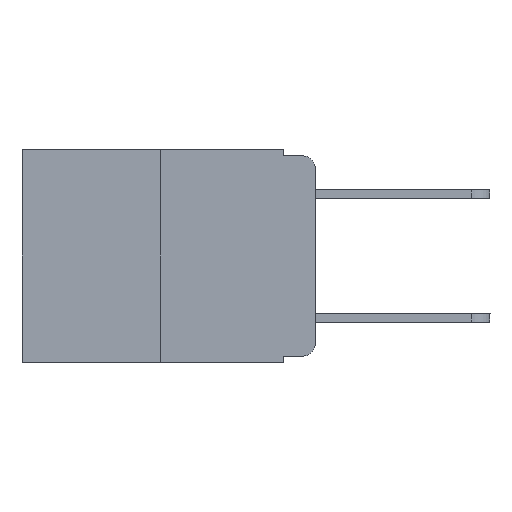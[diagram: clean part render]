
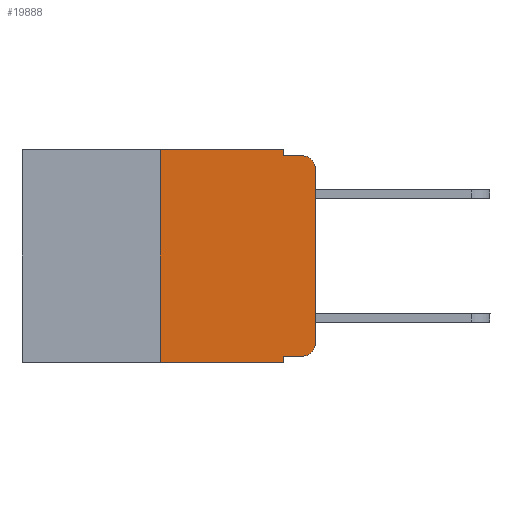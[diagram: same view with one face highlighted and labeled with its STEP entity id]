
A CAD part, left-side view. The second image highlights one B-rep face of the part: STEP entity #19888.
In plain terms, the highlighted planar face has unit normal (-1, 0, 0).
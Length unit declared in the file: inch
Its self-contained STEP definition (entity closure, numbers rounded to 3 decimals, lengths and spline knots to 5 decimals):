
#262 = VECTOR ( 'NONE', #478, 39.37008 ) ;
#307 = VECTOR ( 'NONE', #18379, 39.37008 ) ;
#478 = DIRECTION ( 'NONE',  ( 0., -1., 0. ) ) ;
#493 = DIRECTION ( 'NONE',  ( 0., 0., 1. ) ) ;
#509 = VECTOR ( 'NONE', #14346, 39.37008 ) ;
#698 = DIRECTION ( 'NONE',  ( 0., 0., -1. ) ) ;
#1296 = CARTESIAN_POINT ( 'NONE',  ( 0., 0.25, -0.343 ) ) ;
#1331 = CARTESIAN_POINT ( 'NONE',  ( 0., 0.051, 0. ) ) ;
#1610 = CIRCLE ( 'NONE', #6613, 0.02 ) ;
#1802 = VECTOR ( 'NONE', #15752, 39.37008 ) ;
#1815 = VECTOR ( 'NONE', #493, 39.37008 ) ;
#1986 = CARTESIAN_POINT ( 'NONE',  ( 0., 0.25, 0. ) ) ;
#2283 = CARTESIAN_POINT ( 'NONE',  ( 0., 0.02, -0.313 ) ) ;
#2319 = EDGE_CURVE ( 'NONE', #7240, #7508, #14245, .T. ) ;
#2642 = VERTEX_POINT ( 'NONE', #18880 ) ;
#3036 = ORIENTED_EDGE ( 'NONE', *, *, #4214, .F. ) ;
#3186 = CARTESIAN_POINT ( 'NONE',  ( 0., 0.473, -0.343 ) ) ;
#3391 = EDGE_LOOP ( 'NONE', ( #9204, #11643, #16425, #6075, #3036, #12622, #13894, #13338, #7596, #8342 ) ) ;
#3430 = EDGE_CURVE ( 'NONE', #6850, #14816, #12188, .T. ) ;
#3579 = VECTOR ( 'NONE', #698, 39.37008 ) ;
#3724 = LINE ( 'NONE', #6735, #509 ) ;
#3794 = LINE ( 'NONE', #6949, #1815 ) ;
#4214 = EDGE_CURVE ( 'NONE', #2642, #6850, #18089, .T. ) ;
#4427 = LINE ( 'NONE', #1986, #11347 ) ;
#5440 = EDGE_CURVE ( 'NONE', #14863, #7508, #12551, .T. ) ;
#5442 = CARTESIAN_POINT ( 'NONE',  ( 0., 0.473, 0. ) ) ;
#6024 = LINE ( 'NONE', #13960, #1802 ) ;
#6075 = ORIENTED_EDGE ( 'NONE', *, *, #3430, .F. ) ;
#6363 = AXIS2_PLACEMENT_3D ( 'NONE', #9629, #11213, #16265 ) ;
#6613 = AXIS2_PLACEMENT_3D ( 'NONE', #13531, #13325, #10352 ) ;
#6735 = CARTESIAN_POINT ( 'NONE',  ( 0., 0.051, -0.333 ) ) ;
#6784 = DIRECTION ( 'NONE',  ( 0., 0., 1. ) ) ;
#6850 = VERTEX_POINT ( 'NONE', #1331 ) ;
#6949 = CARTESIAN_POINT ( 'NONE',  ( 0., 0., 0. ) ) ;
#7031 = DIRECTION ( 'NONE',  ( 0., 0., -1. ) ) ;
#7192 = CARTESIAN_POINT ( 'NONE',  ( 0., 0.051, -0.01 ) ) ;
#7240 = VERTEX_POINT ( 'NONE', #17338 ) ;
#7508 = VERTEX_POINT ( 'NONE', #12975 ) ;
#7596 = ORIENTED_EDGE ( 'NONE', *, *, #15101, .T. ) ;
#8056 = PLANE ( 'NONE',  #6363 ) ;
#8342 = ORIENTED_EDGE ( 'NONE', *, *, #10342, .T. ) ;
#8515 = FACE_OUTER_BOUND ( 'NONE', #3391, .T. ) ;
#8824 = EDGE_CURVE ( 'NONE', #14816, #16601, #6024, .T. ) ;
#9204 = ORIENTED_EDGE ( 'NONE', *, *, #19451, .T. ) ;
#9629 = CARTESIAN_POINT ( 'NONE',  ( 0., 0.473, 0. ) ) ;
#10342 = EDGE_CURVE ( 'NONE', #18306, #12834, #19798, .T. ) ;
#10352 = DIRECTION ( 'NONE',  ( 0., 0., -1. ) ) ;
#10446 = CARTESIAN_POINT ( 'NONE',  ( 0., 0.02, -0.333 ) ) ;
#10887 = VERTEX_POINT ( 'NONE', #13364 ) ;
#11213 = DIRECTION ( 'NONE',  ( 1., 0., 0. ) ) ;
#11347 = VECTOR ( 'NONE', #6784, 39.37008 ) ;
#11643 = ORIENTED_EDGE ( 'NONE', *, *, #18905, .T. ) ;
#11684 = CARTESIAN_POINT ( 'NONE',  ( 0., 0., -0.313 ) ) ;
#12188 = LINE ( 'NONE', #13615, #307 ) ;
#12551 = LINE ( 'NONE', #3186, #18969 ) ;
#12622 = ORIENTED_EDGE ( 'NONE', *, *, #16501, .F. ) ;
#12707 = AXIS2_PLACEMENT_3D ( 'NONE', #2283, #14772, #7031 ) ;
#12834 = VERTEX_POINT ( 'NONE', #11684 ) ;
#12975 = CARTESIAN_POINT ( 'NONE',  ( 0., 0.051, -0.343 ) ) ;
#13325 = DIRECTION ( 'NONE',  ( -1., 0., 0. ) ) ;
#13338 = ORIENTED_EDGE ( 'NONE', *, *, #2319, .F. ) ;
#13364 = CARTESIAN_POINT ( 'NONE',  ( 0., 0., -0.03 ) ) ;
#13531 = CARTESIAN_POINT ( 'NONE',  ( 0., 0.02, -0.03 ) ) ;
#13615 = CARTESIAN_POINT ( 'NONE',  ( 0., 0.051, 0. ) ) ;
#13894 = ORIENTED_EDGE ( 'NONE', *, *, #5440, .T. ) ;
#13960 = CARTESIAN_POINT ( 'NONE',  ( 0., 0.051, -0.01 ) ) ;
#14245 = LINE ( 'NONE', #17981, #3579 ) ;
#14269 = DIRECTION ( 'NONE',  ( 0., -1., 0. ) ) ;
#14346 = DIRECTION ( 'NONE',  ( 0., -1., 0. ) ) ;
#14772 = DIRECTION ( 'NONE',  ( -1., 0., 0. ) ) ;
#14816 = VERTEX_POINT ( 'NONE', #7192 ) ;
#14863 = VERTEX_POINT ( 'NONE', #1296 ) ;
#15101 = EDGE_CURVE ( 'NONE', #7240, #18306, #3724, .T. ) ;
#15273 = CARTESIAN_POINT ( 'NONE',  ( 0., 0.02, -0.01 ) ) ;
#15752 = DIRECTION ( 'NONE',  ( 0., -1., 0. ) ) ;
#16265 = DIRECTION ( 'NONE',  ( 0., 0., -1. ) ) ;
#16425 = ORIENTED_EDGE ( 'NONE', *, *, #8824, .F. ) ;
#16501 = EDGE_CURVE ( 'NONE', #14863, #2642, #4427, .T. ) ;
#16601 = VERTEX_POINT ( 'NONE', #15273 ) ;
#17338 = CARTESIAN_POINT ( 'NONE',  ( 0., 0.051, -0.333 ) ) ;
#17981 = CARTESIAN_POINT ( 'NONE',  ( 0., 0.051, 0. ) ) ;
#18089 = LINE ( 'NONE', #5442, #262 ) ;
#18306 = VERTEX_POINT ( 'NONE', #10446 ) ;
#18379 = DIRECTION ( 'NONE',  ( 0., 0., -1. ) ) ;
#18880 = CARTESIAN_POINT ( 'NONE',  ( 0., 0.25, 0. ) ) ;
#18905 = EDGE_CURVE ( 'NONE', #10887, #16601, #1610, .T. ) ;
#18969 = VECTOR ( 'NONE', #14269, 39.37008 ) ;
#19451 = EDGE_CURVE ( 'NONE', #12834, #10887, #3794, .T. ) ;
#19798 = CIRCLE ( 'NONE', #12707, 0.02 ) ;
#19888 = ADVANCED_FACE ( 'NONE', ( #8515 ), #8056, .F. ) ;
